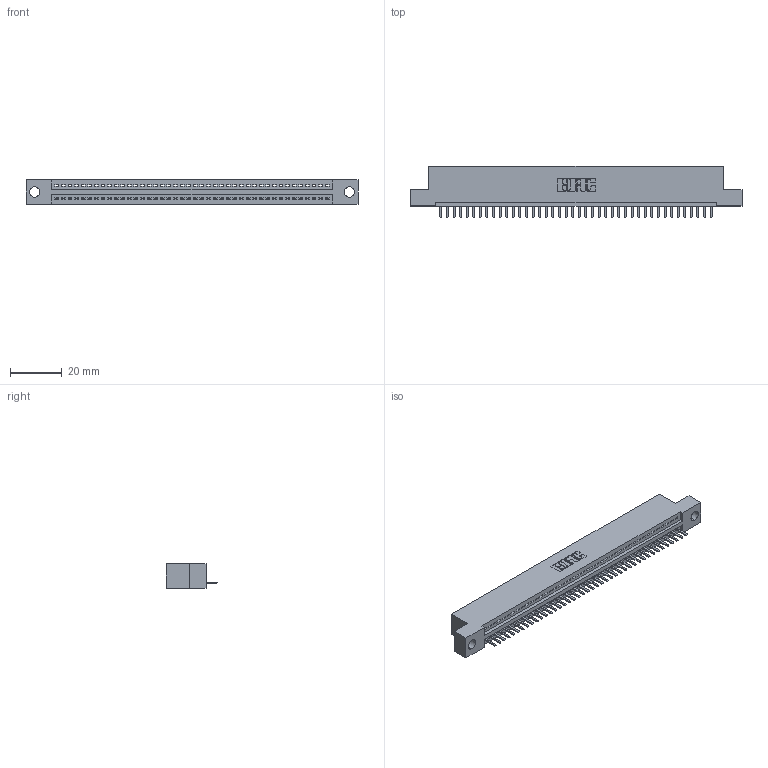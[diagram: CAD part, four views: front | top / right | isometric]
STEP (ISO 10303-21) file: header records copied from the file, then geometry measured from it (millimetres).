
FILE_DESCRIPTION (( 'STEP AP203' ), '1' );
FILE_NAME ('345-042-520-104.STEP', '2021-05-26T15:01:28', ( '' ), ( '' ), 'SwSTEP 2.0', 'SolidWorks 2020', '' );
FILE_SCHEMA (( 'CONFIG_CONTROL_DESIGN' ));
Length unit declared in the file: inch
Products named in the file (3): 345 Part_Flush Mounting Lugs - 0.156 Dia-TI; 345-292-001_345-293-120; 345-042-520-104
Assembly tree (43 placements, depth 2):
  345-042-520-104
    345 Part_Flush Mounting Lugs - 0.156 Dia-TI
    345-292-001_345-293-120  x42
Bounding box: 127.89 x 19.68 x 9.4 mm (x, y, z)
Volume: 11920.3 mm3; surface area: 15288.2 mm2
Topology: 43 solids, 43 shells, 2744 faces, 8105 edges, 5290 vertices
Faces by surface type: plane 1858, cylinder 886
Entity records: 32143 total; most frequent: CARTESIAN_POINT 5588, ORIENTED_EDGE 5550, DIRECTION 4867, EDGE_CURVE 2775, LINE 2471, VECTOR 2471, VERTEX_POINT 1846, AXIS2_PLACEMENT_3D 1198
